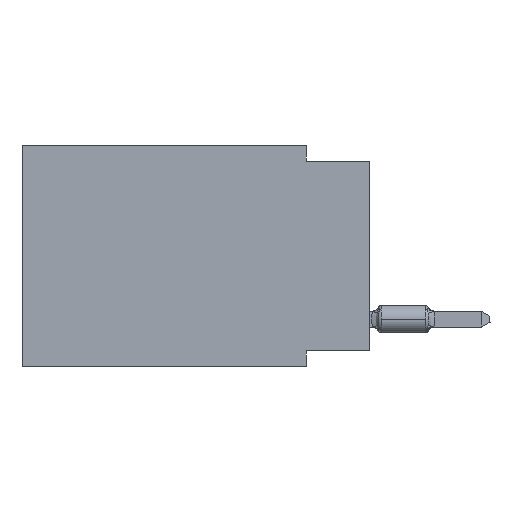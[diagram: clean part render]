
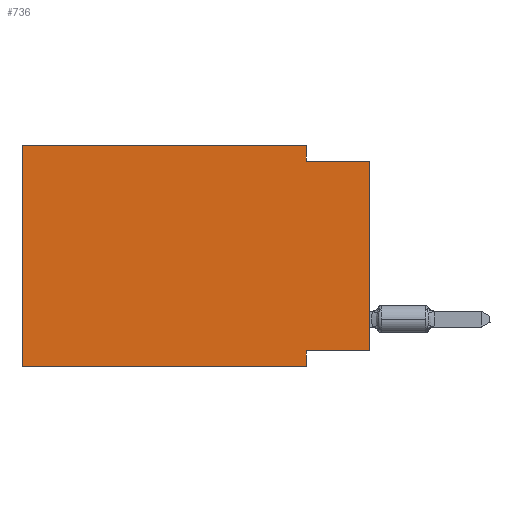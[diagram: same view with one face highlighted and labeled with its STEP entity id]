
A CAD part, left-side view. The second image highlights one B-rep face of the part: STEP entity #736.
In plain terms, the highlighted planar face has unit normal (-1, 0, 0).
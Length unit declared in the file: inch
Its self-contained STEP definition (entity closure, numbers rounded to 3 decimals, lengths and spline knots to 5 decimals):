
#100 = LINE ( 'NONE', #19449, #12969 ) ;
#736 = ADVANCED_FACE ( 'NONE', ( #14318 ), #29139, .F. ) ;
#1155 = VERTEX_POINT ( 'NONE', #17023 ) ;
#1200 = VERTEX_POINT ( 'NONE', #5253 ) ;
#1676 = VERTEX_POINT ( 'NONE', #5211 ) ;
#2243 = EDGE_CURVE ( 'NONE', #19911, #34297, #35878, .T. ) ;
#3613 = EDGE_CURVE ( 'NONE', #1200, #1155, #27904, .T. ) ;
#4616 = EDGE_CURVE ( 'NONE', #1676, #30014, #100, .T. ) ;
#4863 = DIRECTION ( 'NONE',  ( 0., 0., 1. ) ) ;
#5038 = DIRECTION ( 'NONE',  ( 0., 1., 0. ) ) ;
#5211 = CARTESIAN_POINT ( 'NONE',  ( 0., 0., -0.325 ) ) ;
#5253 = CARTESIAN_POINT ( 'NONE',  ( 0., 0.1, -0.025 ) ) ;
#6136 = VECTOR ( 'NONE', #14826, 39.37008 ) ;
#7137 = VECTOR ( 'NONE', #28702, 39.37008 ) ;
#8096 = LINE ( 'NONE', #33706, #20485 ) ;
#8196 = DIRECTION ( 'NONE',  ( 0., 0., -1. ) ) ;
#8580 = VECTOR ( 'NONE', #37540, 39.37008 ) ;
#8709 = CARTESIAN_POINT ( 'NONE',  ( 0., 0.55, 0. ) ) ;
#9131 = VERTEX_POINT ( 'NONE', #26990 ) ;
#10059 = ORIENTED_EDGE ( 'NONE', *, *, #25445, .F. ) ;
#11036 = LINE ( 'NONE', #22607, #36313 ) ;
#12721 = ORIENTED_EDGE ( 'NONE', *, *, #20242, .T. ) ;
#12969 = VECTOR ( 'NONE', #5038, 39.37008 ) ;
#14318 = FACE_OUTER_BOUND ( 'NONE', #35846, .T. ) ;
#14826 = DIRECTION ( 'NONE',  ( 0., 0., 1. ) ) ;
#16102 = ORIENTED_EDGE ( 'NONE', *, *, #4616, .F. ) ;
#17023 = CARTESIAN_POINT ( 'NONE',  ( 0., 0., -0.025 ) ) ;
#17053 = LINE ( 'NONE', #8709, #8580 ) ;
#17122 = LINE ( 'NONE', #22243, #7137 ) ;
#17356 = DIRECTION ( 'NONE',  ( 1., 0., 0. ) ) ;
#17669 = CARTESIAN_POINT ( 'NONE',  ( 0., 0.55, -0.35 ) ) ;
#19198 = VERTEX_POINT ( 'NONE', #30627 ) ;
#19449 = CARTESIAN_POINT ( 'NONE',  ( 0., 0., -0.325 ) ) ;
#19819 = DIRECTION ( 'NONE',  ( 0., 0., -1. ) ) ;
#19911 = VERTEX_POINT ( 'NONE', #17669 ) ;
#20242 = EDGE_CURVE ( 'NONE', #1676, #1155, #8096, .T. ) ;
#20305 = DIRECTION ( 'NONE',  ( 0., -1., 0. ) ) ;
#20485 = VECTOR ( 'NONE', #4863, 39.37008 ) ;
#22243 = CARTESIAN_POINT ( 'NONE',  ( 0., 0.1, -0.35 ) ) ;
#22607 = CARTESIAN_POINT ( 'NONE',  ( 0., 0.1, 0. ) ) ;
#23055 = CARTESIAN_POINT ( 'NONE',  ( 0., 0.55, 0. ) ) ;
#23517 = CARTESIAN_POINT ( 'NONE',  ( 0., 0.55, -0.35 ) ) ;
#23549 = CARTESIAN_POINT ( 'NONE',  ( 0., 0.55, 0. ) ) ;
#24849 = ORIENTED_EDGE ( 'NONE', *, *, #32496, .F. ) ;
#25424 = CARTESIAN_POINT ( 'NONE',  ( 0., 0., -0.025 ) ) ;
#25445 = EDGE_CURVE ( 'NONE', #34297, #19198, #17053, .T. ) ;
#26990 = CARTESIAN_POINT ( 'NONE',  ( 0., 0.1, -0.35 ) ) ;
#27088 = ORIENTED_EDGE ( 'NONE', *, *, #32980, .T. ) ;
#27869 = VECTOR ( 'NONE', #30558, 39.37008 ) ;
#27904 = LINE ( 'NONE', #25424, #27869 ) ;
#27913 = EDGE_CURVE ( 'NONE', #19198, #1200, #11036, .T. ) ;
#28702 = DIRECTION ( 'NONE',  ( 0., 0., -1. ) ) ;
#29139 = PLANE ( 'NONE',  #33312 ) ;
#29197 = VECTOR ( 'NONE', #20305, 39.37008 ) ;
#29380 = ORIENTED_EDGE ( 'NONE', *, *, #27913, .F. ) ;
#29775 = CARTESIAN_POINT ( 'NONE',  ( 0., 0.55, 0. ) ) ;
#30014 = VERTEX_POINT ( 'NONE', #30771 ) ;
#30558 = DIRECTION ( 'NONE',  ( 0., -1., 0. ) ) ;
#30627 = CARTESIAN_POINT ( 'NONE',  ( 0., 0.1, 0. ) ) ;
#30771 = CARTESIAN_POINT ( 'NONE',  ( 0., 0.1, -0.325 ) ) ;
#32255 = LINE ( 'NONE', #23517, #29197 ) ;
#32496 = EDGE_CURVE ( 'NONE', #30014, #9131, #17122, .T. ) ;
#32980 = EDGE_CURVE ( 'NONE', #19911, #9131, #32255, .T. ) ;
#33312 = AXIS2_PLACEMENT_3D ( 'NONE', #23055, #17356, #19819 ) ;
#33706 = CARTESIAN_POINT ( 'NONE',  ( 0., 0., 0. ) ) ;
#34297 = VERTEX_POINT ( 'NONE', #29775 ) ;
#35785 = ORIENTED_EDGE ( 'NONE', *, *, #2243, .F. ) ;
#35846 = EDGE_LOOP ( 'NONE', ( #12721, #37368, #29380, #10059, #35785, #27088, #24849, #16102 ) ) ;
#35878 = LINE ( 'NONE', #23549, #6136 ) ;
#36313 = VECTOR ( 'NONE', #8196, 39.37008 ) ;
#37368 = ORIENTED_EDGE ( 'NONE', *, *, #3613, .F. ) ;
#37540 = DIRECTION ( 'NONE',  ( 0., -1., 0. ) ) ;
